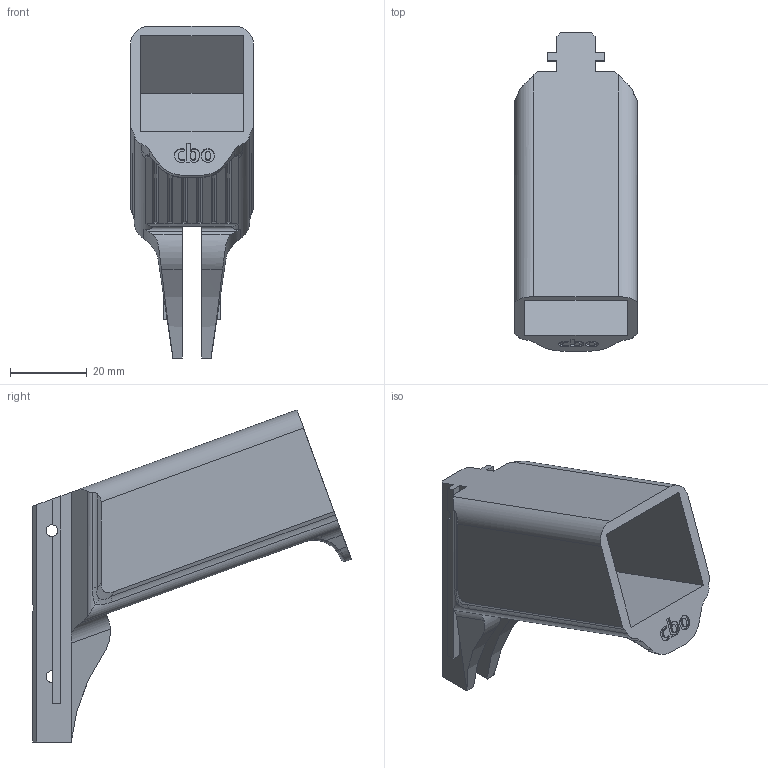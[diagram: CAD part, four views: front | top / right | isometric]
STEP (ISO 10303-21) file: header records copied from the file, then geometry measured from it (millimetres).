
FILE_DESCRIPTION (( 'STEP AP214' ), '1' );
FILE_NAME ('LowerGrip^StikM1.STEP', '2013-09-01T22:38:25', ( 'Asher' ), ( '' ), 'SwSTEP 2.0', 'SolidWorks 2013', '' );
FILE_SCHEMA (( 'AUTOMOTIVE_DESIGN' ));
Length unit declared in the file: millimetre
Products named in the file (1): LowerGrip^StikM1
Bounding box: 32 x 82.88 x 86.38 mm (x, y, z)
Volume: 42974.2 mm3; surface area: 19980.3 mm2
Topology: 1 solids, 1 shells, 190 faces, 524 edges, 333 vertices
Faces by surface type: plane 82, cylinder 69, bspline 39
Entity records: 7961 total; most frequent: CARTESIAN_POINT 3574, ORIENTED_EDGE 1040, DIRECTION 725, EDGE_CURVE 520, VERTEX_POINT 333, LINE 297, VECTOR 297, AXIS2_PLACEMENT_3D 214
